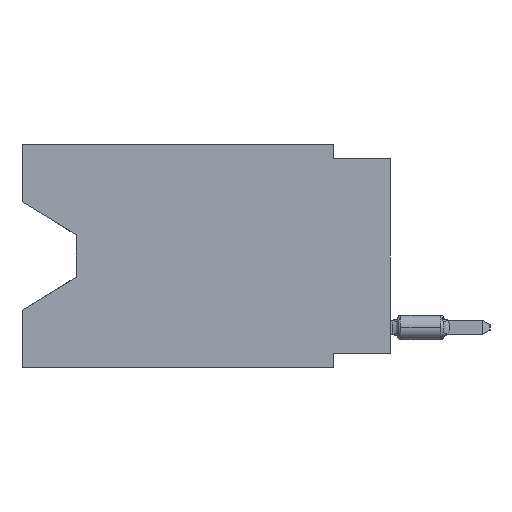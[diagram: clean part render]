
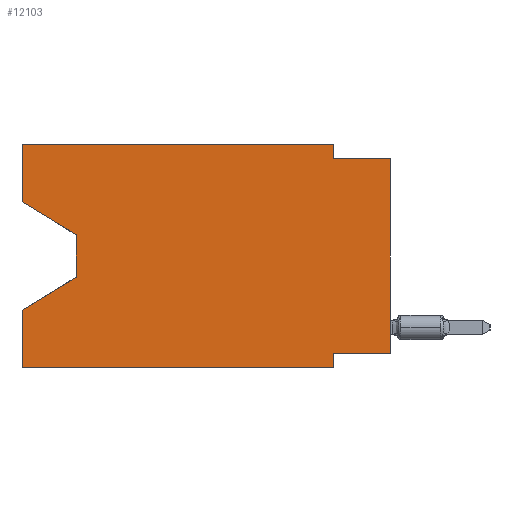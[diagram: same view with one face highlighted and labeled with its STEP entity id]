
A CAD part, left-side view. The second image highlights one B-rep face of the part: STEP entity #12103.
In plain terms, the highlighted planar face has unit normal (-1, 0, 0).
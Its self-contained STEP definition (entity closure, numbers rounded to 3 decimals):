
#179 = VECTOR ( 'NONE', #8008, 1000. ) ;
#219 = VECTOR ( 'NONE', #28992, 1000. ) ;
#589 = CARTESIAN_POINT ( 'NONE',  ( 0., 0., -0.635 ) ) ;
#937 = LINE ( 'NONE', #12999, #22171 ) ;
#1339 = VECTOR ( 'NONE', #21326, 1000. ) ;
#2100 = EDGE_CURVE ( 'NONE', #21852, #16482, #8090, .T. ) ;
#2529 = LINE ( 'NONE', #18640, #28811 ) ;
#2780 = AXIS2_PLACEMENT_3D ( 'NONE', #8038, #17303, #26757 ) ;
#2787 = EDGE_CURVE ( 'NONE', #30233, #6430, #19182, .T. ) ;
#2971 = ORIENTED_EDGE ( 'NONE', *, *, #10348, .F. ) ;
#3152 = VERTEX_POINT ( 'NONE', #19217 ) ;
#3529 = VECTOR ( 'NONE', #17514, 1000. ) ;
#3625 = CARTESIAN_POINT ( 'NONE',  ( 0., 2.54, -0.635 ) ) ;
#4047 = LINE ( 'NONE', #30361, #5819 ) ;
#4337 = EDGE_LOOP ( 'NONE', ( #6700, #10509, #14346, #10152, #16138, #5314, #10241, #7275, #17799, #27603, #25496, #2971 ) ) ;
#4468 = DIRECTION ( 'NONE',  ( 0., 0., -1. ) ) ;
#4606 = CARTESIAN_POINT ( 'NONE',  ( 0., 16.383, -9.906 ) ) ;
#4893 = EDGE_CURVE ( 'NONE', #3152, #30233, #4047, .T. ) ;
#5128 = LINE ( 'NONE', #17637, #19444 ) ;
#5314 = ORIENTED_EDGE ( 'NONE', *, *, #9709, .F. ) ;
#5538 = CARTESIAN_POINT ( 'NONE',  ( 0., 0., -9.271 ) ) ;
#5819 = VECTOR ( 'NONE', #20615, 1000. ) ;
#5957 = CARTESIAN_POINT ( 'NONE',  ( 0., 13.97, -5.893 ) ) ;
#6430 = VERTEX_POINT ( 'NONE', #589 ) ;
#6700 = ORIENTED_EDGE ( 'NONE', *, *, #2100, .T. ) ;
#7275 = ORIENTED_EDGE ( 'NONE', *, *, #15446, .T. ) ;
#7877 = FACE_OUTER_BOUND ( 'NONE', #4337, .T. ) ;
#8008 = DIRECTION ( 'NONE',  ( 0., 1., 0. ) ) ;
#8038 = CARTESIAN_POINT ( 'NONE',  ( 0., 16.383, 0. ) ) ;
#8090 = LINE ( 'NONE', #13034, #219 ) ;
#8163 = CARTESIAN_POINT ( 'NONE',  ( 0., 13.97, -4.013 ) ) ;
#8897 = LINE ( 'NONE', #29798, #15024 ) ;
#9709 = EDGE_CURVE ( 'NONE', #29063, #25041, #27685, .T. ) ;
#10152 = ORIENTED_EDGE ( 'NONE', *, *, #14932, .F. ) ;
#10241 = ORIENTED_EDGE ( 'NONE', *, *, #16129, .F. ) ;
#10348 = EDGE_CURVE ( 'NONE', #21852, #21437, #29142, .T. ) ;
#10509 = ORIENTED_EDGE ( 'NONE', *, *, #24112, .T. ) ;
#10939 = VERTEX_POINT ( 'NONE', #12827 ) ;
#11275 = CARTESIAN_POINT ( 'NONE',  ( 0., 2.54, -9.906 ) ) ;
#11897 = VECTOR ( 'NONE', #4468, 1000. ) ;
#12103 = ADVANCED_FACE ( 'NONE', ( #7877 ), #29407, .F. ) ;
#12493 = CARTESIAN_POINT ( 'NONE',  ( 0., 16.383, -2.546 ) ) ;
#12827 = CARTESIAN_POINT ( 'NONE',  ( 0., 16.383, -7.36 ) ) ;
#12882 = DIRECTION ( 'NONE',  ( 0., 0., 1. ) ) ;
#12999 = CARTESIAN_POINT ( 'NONE',  ( 0., 16.383, 0. ) ) ;
#13034 = CARTESIAN_POINT ( 'NONE',  ( 0., 16.383, -2.546 ) ) ;
#13754 = DIRECTION ( 'NONE',  ( 0., 0., -1. ) ) ;
#14055 = CARTESIAN_POINT ( 'NONE',  ( 0., 0., -0.635 ) ) ;
#14346 = ORIENTED_EDGE ( 'NONE', *, *, #20198, .T. ) ;
#14862 = EDGE_CURVE ( 'NONE', #26025, #25041, #2529, .T. ) ;
#14932 = EDGE_CURVE ( 'NONE', #26025, #10939, #19403, .T. ) ;
#15024 = VECTOR ( 'NONE', #27333, 1000. ) ;
#15176 = CARTESIAN_POINT ( 'NONE',  ( 0., 0., -9.271 ) ) ;
#15446 = EDGE_CURVE ( 'NONE', #17219, #6430, #5128, .T. ) ;
#16074 = CARTESIAN_POINT ( 'NONE',  ( 0., 13.97, -4.013 ) ) ;
#16129 = EDGE_CURVE ( 'NONE', #17219, #29063, #27358, .T. ) ;
#16138 = ORIENTED_EDGE ( 'NONE', *, *, #14862, .T. ) ;
#16482 = VERTEX_POINT ( 'NONE', #8163 ) ;
#17219 = VERTEX_POINT ( 'NONE', #15176 ) ;
#17303 = DIRECTION ( 'NONE',  ( 1., 0., 0. ) ) ;
#17323 = DIRECTION ( 'NONE',  ( 0., -1., 0. ) ) ;
#17514 = DIRECTION ( 'NONE',  ( 0., 0., 1. ) ) ;
#17637 = CARTESIAN_POINT ( 'NONE',  ( 0., 0., 0. ) ) ;
#17717 = VECTOR ( 'NONE', #13754, 1000. ) ;
#17799 = ORIENTED_EDGE ( 'NONE', *, *, #2787, .F. ) ;
#18640 = CARTESIAN_POINT ( 'NONE',  ( 0., 16.383, -9.906 ) ) ;
#19182 = LINE ( 'NONE', #14055, #1339 ) ;
#19217 = CARTESIAN_POINT ( 'NONE',  ( 0., 2.54, 0. ) ) ;
#19403 = LINE ( 'NONE', #26516, #23382 ) ;
#19444 = VECTOR ( 'NONE', #19977, 1000. ) ;
#19977 = DIRECTION ( 'NONE',  ( 0., 0., 1. ) ) ;
#20124 = CARTESIAN_POINT ( 'NONE',  ( 0., 16.383, 0. ) ) ;
#20198 = EDGE_CURVE ( 'NONE', #20632, #10939, #8897, .T. ) ;
#20585 = LINE ( 'NONE', #16074, #17717 ) ;
#20615 = DIRECTION ( 'NONE',  ( 0., 0., -1. ) ) ;
#20632 = VERTEX_POINT ( 'NONE', #5957 ) ;
#21111 = DIRECTION ( 'NONE',  ( 0., -1., 0. ) ) ;
#21326 = DIRECTION ( 'NONE',  ( 0., -1., 0. ) ) ;
#21437 = VERTEX_POINT ( 'NONE', #20124 ) ;
#21852 = VERTEX_POINT ( 'NONE', #12493 ) ;
#22021 = CARTESIAN_POINT ( 'NONE',  ( 0., 16.383, 0. ) ) ;
#22171 = VECTOR ( 'NONE', #17323, 1000. ) ;
#22517 = CARTESIAN_POINT ( 'NONE',  ( 0., 2.54, -9.271 ) ) ;
#23382 = VECTOR ( 'NONE', #12882, 1000. ) ;
#23996 = EDGE_CURVE ( 'NONE', #21437, #3152, #937, .T. ) ;
#24112 = EDGE_CURVE ( 'NONE', #16482, #20632, #20585, .T. ) ;
#25041 = VERTEX_POINT ( 'NONE', #28812 ) ;
#25496 = ORIENTED_EDGE ( 'NONE', *, *, #23996, .F. ) ;
#26025 = VERTEX_POINT ( 'NONE', #4606 ) ;
#26516 = CARTESIAN_POINT ( 'NONE',  ( 0., 16.383, 0. ) ) ;
#26757 = DIRECTION ( 'NONE',  ( 0., 0., -1. ) ) ;
#27333 = DIRECTION ( 'NONE',  ( 0., 0.855, -0.519 ) ) ;
#27358 = LINE ( 'NONE', #5538, #179 ) ;
#27603 = ORIENTED_EDGE ( 'NONE', *, *, #4893, .F. ) ;
#27685 = LINE ( 'NONE', #11275, #11897 ) ;
#28811 = VECTOR ( 'NONE', #21111, 1000. ) ;
#28812 = CARTESIAN_POINT ( 'NONE',  ( 0., 2.54, -9.906 ) ) ;
#28992 = DIRECTION ( 'NONE',  ( 0., -0.855, -0.519 ) ) ;
#29063 = VERTEX_POINT ( 'NONE', #22517 ) ;
#29142 = LINE ( 'NONE', #22021, #3529 ) ;
#29407 = PLANE ( 'NONE',  #2780 ) ;
#29798 = CARTESIAN_POINT ( 'NONE',  ( 0., 13.97, -5.893 ) ) ;
#30233 = VERTEX_POINT ( 'NONE', #3625 ) ;
#30361 = CARTESIAN_POINT ( 'NONE',  ( 0., 2.54, 0. ) ) ;
